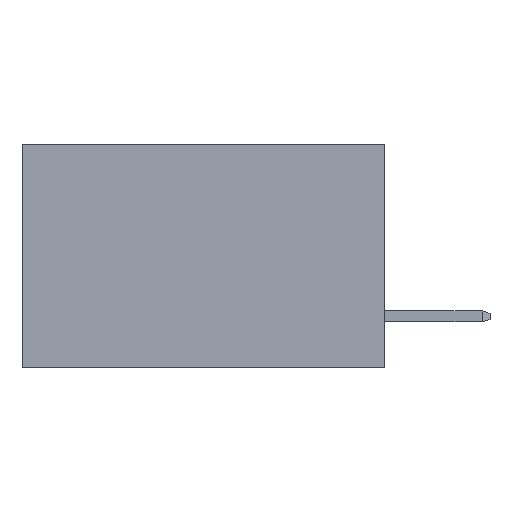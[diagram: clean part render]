
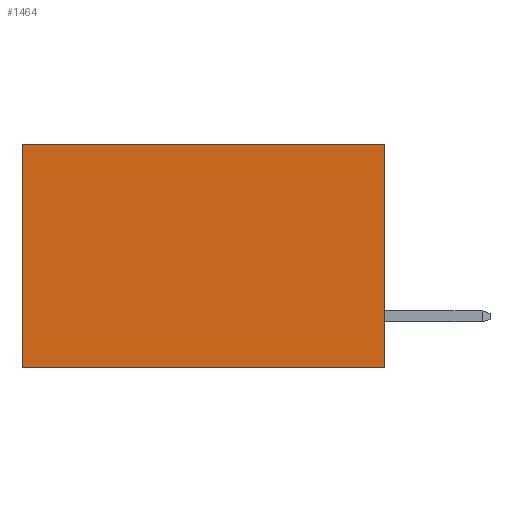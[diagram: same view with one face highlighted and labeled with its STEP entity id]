
A CAD part, left-side view. The second image highlights one B-rep face of the part: STEP entity #1464.
In plain terms, the highlighted planar face has unit normal (-1, 0, 0).
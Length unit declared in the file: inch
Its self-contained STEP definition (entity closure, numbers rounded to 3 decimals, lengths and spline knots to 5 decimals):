
#162 = DIRECTION ( 'NONE',  ( 1., 0., 0. ) ) ;
#224 = DIRECTION ( 'NONE',  ( 0., 0., -1. ) ) ;
#318 = VECTOR ( 'NONE', #7398, 39.37008 ) ;
#341 = VERTEX_POINT ( 'NONE', #5418 ) ;
#453 = CARTESIAN_POINT ( 'NONE',  ( 0.2615, 0., 0. ) ) ;
#536 = LINE ( 'NONE', #7439, #318 ) ;
#912 = EDGE_CURVE ( 'NONE', #2153, #341, #6107, .T. ) ;
#1355 = ORIENTED_EDGE ( 'NONE', *, *, #3549, .F. ) ;
#1464 = ADVANCED_FACE ( 'NONE', ( #6385 ), #7711, .F. ) ;
#1647 = CARTESIAN_POINT ( 'NONE',  ( 0.2615, 0.6, -0.37 ) ) ;
#1801 = DIRECTION ( 'NONE',  ( 0., 0., -1. ) ) ;
#2153 = VERTEX_POINT ( 'NONE', #4892 ) ;
#2560 = ORIENTED_EDGE ( 'NONE', *, *, #6484, .T. ) ;
#3348 = CARTESIAN_POINT ( 'NONE',  ( 0.2615, 0., -0.37 ) ) ;
#3422 = DIRECTION ( 'NONE',  ( 0., 1., 0. ) ) ;
#3549 = EDGE_CURVE ( 'NONE', #3693, #341, #5978, .T. ) ;
#3686 = CARTESIAN_POINT ( 'NONE',  ( 0.2615, 0., -0.37 ) ) ;
#3693 = VERTEX_POINT ( 'NONE', #8547 ) ;
#3769 = EDGE_LOOP ( 'NONE', ( #5888, #1355, #5693, #2560 ) ) ;
#3835 = DIRECTION ( 'NONE',  ( 0., 0., -1. ) ) ;
#4193 = CARTESIAN_POINT ( 'NONE',  ( 0.2615, 0., -0.37 ) ) ;
#4368 = VECTOR ( 'NONE', #1801, 39.37008 ) ;
#4892 = CARTESIAN_POINT ( 'NONE',  ( 0.2615, 0.6, 0. ) ) ;
#5355 = LINE ( 'NONE', #3686, #7052 ) ;
#5418 = CARTESIAN_POINT ( 'NONE',  ( 0.2615, 0.6, -0.37 ) ) ;
#5693 = ORIENTED_EDGE ( 'NONE', *, *, #6931, .F. ) ;
#5781 = VECTOR ( 'NONE', #3422, 39.37008 ) ;
#5840 = AXIS2_PLACEMENT_3D ( 'NONE', #4193, #162, #224 ) ;
#5849 = VERTEX_POINT ( 'NONE', #453 ) ;
#5888 = ORIENTED_EDGE ( 'NONE', *, *, #912, .T. ) ;
#5978 = LINE ( 'NONE', #3348, #5781 ) ;
#6107 = LINE ( 'NONE', #1647, #4368 ) ;
#6385 = FACE_OUTER_BOUND ( 'NONE', #3769, .T. ) ;
#6484 = EDGE_CURVE ( 'NONE', #5849, #2153, #536, .T. ) ;
#6931 = EDGE_CURVE ( 'NONE', #5849, #3693, #5355, .T. ) ;
#7052 = VECTOR ( 'NONE', #3835, 39.37008 ) ;
#7398 = DIRECTION ( 'NONE',  ( 0., 1., 0. ) ) ;
#7439 = CARTESIAN_POINT ( 'NONE',  ( 0.2615, 0., 0. ) ) ;
#7711 = PLANE ( 'NONE',  #5840 ) ;
#8547 = CARTESIAN_POINT ( 'NONE',  ( 0.2615, 0., -0.37 ) ) ;
